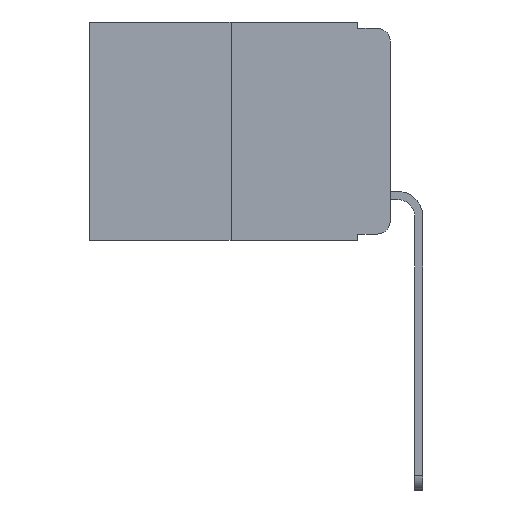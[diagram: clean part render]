
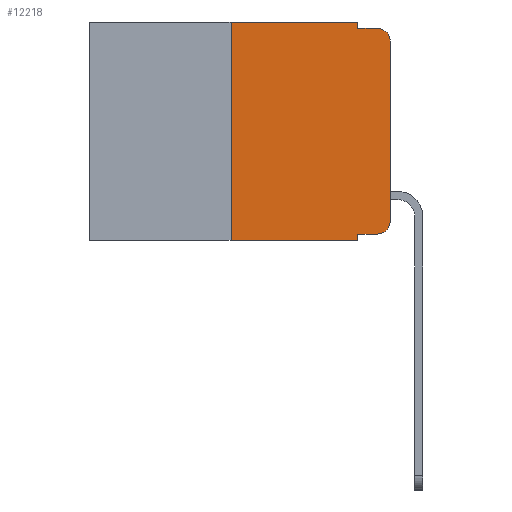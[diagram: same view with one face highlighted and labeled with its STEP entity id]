
A CAD part, left-side view. The second image highlights one B-rep face of the part: STEP entity #12218.
In plain terms, the highlighted planar face has unit normal (-1, 0, 0).
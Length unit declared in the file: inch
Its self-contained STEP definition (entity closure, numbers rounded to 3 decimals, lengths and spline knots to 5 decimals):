
#92 = CARTESIAN_POINT ( 'NONE',  ( 0., 0.25, -0.343 ) ) ;
#137 = VERTEX_POINT ( 'NONE', #10585 ) ;
#212 = EDGE_CURVE ( 'NONE', #8192, #11914, #12393, .T. ) ;
#644 = ORIENTED_EDGE ( 'NONE', *, *, #1718, .F. ) ;
#750 = CIRCLE ( 'NONE', #8688, 0.02 ) ;
#809 = DIRECTION ( 'NONE',  ( 0., 0., -1. ) ) ;
#830 = LINE ( 'NONE', #10785, #11550 ) ;
#1185 = CARTESIAN_POINT ( 'NONE',  ( 0., 0.051, -0.01 ) ) ;
#1364 = ORIENTED_EDGE ( 'NONE', *, *, #6208, .T. ) ;
#1379 = CARTESIAN_POINT ( 'NONE',  ( 0., 0.051, -0.333 ) ) ;
#1653 = EDGE_CURVE ( 'NONE', #8192, #5656, #4548, .T. ) ;
#1718 = EDGE_CURVE ( 'NONE', #12948, #137, #2515, .T. ) ;
#1779 = EDGE_CURVE ( 'NONE', #12948, #11914, #5555, .T. ) ;
#1780 = LINE ( 'NONE', #13300, #13002 ) ;
#2081 = EDGE_CURVE ( 'NONE', #5454, #8555, #10981, .T. ) ;
#2210 = ORIENTED_EDGE ( 'NONE', *, *, #2878, .T. ) ;
#2274 = DIRECTION ( 'NONE',  ( 0., -1., 0. ) ) ;
#2314 = ORIENTED_EDGE ( 'NONE', *, *, #1653, .T. ) ;
#2515 = LINE ( 'NONE', #4345, #10824 ) ;
#2773 = CARTESIAN_POINT ( 'NONE',  ( 0., 0.02, -0.01 ) ) ;
#2878 = EDGE_CURVE ( 'NONE', #9328, #3279, #750, .T. ) ;
#2961 = EDGE_CURVE ( 'NONE', #5656, #3837, #5689, .T. ) ;
#3122 = AXIS2_PLACEMENT_3D ( 'NONE', #7548, #4167, #13949 ) ;
#3279 = VERTEX_POINT ( 'NONE', #2773 ) ;
#3567 = CARTESIAN_POINT ( 'NONE',  ( 0., 0.473, 0. ) ) ;
#3784 = LINE ( 'NONE', #3567, #4441 ) ;
#3796 = ORIENTED_EDGE ( 'NONE', *, *, #2081, .F. ) ;
#3808 = CARTESIAN_POINT ( 'NONE',  ( 0., 0., -0.313 ) ) ;
#3837 = VERTEX_POINT ( 'NONE', #3808 ) ;
#4007 = DIRECTION ( 'NONE',  ( -1., 0., 0. ) ) ;
#4167 = DIRECTION ( 'NONE',  ( 1., 0., 0. ) ) ;
#4345 = CARTESIAN_POINT ( 'NONE',  ( 0., 0.25, 0. ) ) ;
#4377 = CARTESIAN_POINT ( 'NONE',  ( 0., 0.02, -0.333 ) ) ;
#4441 = VECTOR ( 'NONE', #5489, 39.37008 ) ;
#4459 = CARTESIAN_POINT ( 'NONE',  ( 0., 0.051, 0. ) ) ;
#4548 = LINE ( 'NONE', #13065, #8804 ) ;
#5315 = DIRECTION ( 'NONE',  ( 0., 0., -1. ) ) ;
#5454 = VERTEX_POINT ( 'NONE', #8460 ) ;
#5489 = DIRECTION ( 'NONE',  ( 0., -1., 0. ) ) ;
#5555 = LINE ( 'NONE', #11897, #7950 ) ;
#5656 = VERTEX_POINT ( 'NONE', #4377 ) ;
#5689 = CIRCLE ( 'NONE', #11594, 0.02 ) ;
#6059 = EDGE_CURVE ( 'NONE', #137, #5454, #3784, .T. ) ;
#6208 = EDGE_CURVE ( 'NONE', #3837, #9328, #830, .T. ) ;
#6386 = DIRECTION ( 'NONE',  ( -1., 0., 0. ) ) ;
#6430 = DIRECTION ( 'NONE',  ( 0., 0., 1. ) ) ;
#6542 = DIRECTION ( 'NONE',  ( 0., -1., 0. ) ) ;
#6680 = DIRECTION ( 'NONE',  ( 0., -1., 0. ) ) ;
#7548 = CARTESIAN_POINT ( 'NONE',  ( 0., 0.473, 0. ) ) ;
#7591 = EDGE_LOOP ( 'NONE', ( #1364, #2210, #13489, #3796, #13016, #644, #11150, #10753, #2314, #8291 ) ) ;
#7795 = DIRECTION ( 'NONE',  ( 0., 0., -1. ) ) ;
#7950 = VECTOR ( 'NONE', #2274, 39.37008 ) ;
#7951 = CARTESIAN_POINT ( 'NONE',  ( 0., 0., -0.03 ) ) ;
#8192 = VERTEX_POINT ( 'NONE', #1379 ) ;
#8291 = ORIENTED_EDGE ( 'NONE', *, *, #2961, .T. ) ;
#8460 = CARTESIAN_POINT ( 'NONE',  ( 0., 0.051, 0. ) ) ;
#8555 = VERTEX_POINT ( 'NONE', #1185 ) ;
#8688 = AXIS2_PLACEMENT_3D ( 'NONE', #12596, #4007, #809 ) ;
#8804 = VECTOR ( 'NONE', #6542, 39.37008 ) ;
#9328 = VERTEX_POINT ( 'NONE', #7951 ) ;
#9634 = CARTESIAN_POINT ( 'NONE',  ( 0., 0.02, -0.313 ) ) ;
#9770 = PLANE ( 'NONE',  #3122 ) ;
#9882 = FACE_OUTER_BOUND ( 'NONE', #7591, .T. ) ;
#9885 = EDGE_CURVE ( 'NONE', #8555, #3279, #1780, .T. ) ;
#10501 = DIRECTION ( 'NONE',  ( 0., 0., -1. ) ) ;
#10533 = DIRECTION ( 'NONE',  ( 0., 0., 1. ) ) ;
#10585 = CARTESIAN_POINT ( 'NONE',  ( 0., 0.25, 0. ) ) ;
#10753 = ORIENTED_EDGE ( 'NONE', *, *, #212, .F. ) ;
#10778 = CARTESIAN_POINT ( 'NONE',  ( 0., 0.051, 0. ) ) ;
#10785 = CARTESIAN_POINT ( 'NONE',  ( 0., 0., 0. ) ) ;
#10824 = VECTOR ( 'NONE', #6430, 39.37008 ) ;
#10981 = LINE ( 'NONE', #4459, #13877 ) ;
#11150 = ORIENTED_EDGE ( 'NONE', *, *, #1779, .T. ) ;
#11550 = VECTOR ( 'NONE', #10533, 39.37008 ) ;
#11594 = AXIS2_PLACEMENT_3D ( 'NONE', #9634, #6386, #10501 ) ;
#11897 = CARTESIAN_POINT ( 'NONE',  ( 0., 0.473, -0.343 ) ) ;
#11914 = VERTEX_POINT ( 'NONE', #13781 ) ;
#12218 = ADVANCED_FACE ( 'NONE', ( #9882 ), #9770, .F. ) ;
#12393 = LINE ( 'NONE', #10778, #13437 ) ;
#12596 = CARTESIAN_POINT ( 'NONE',  ( 0., 0.02, -0.03 ) ) ;
#12948 = VERTEX_POINT ( 'NONE', #92 ) ;
#13002 = VECTOR ( 'NONE', #6680, 39.37008 ) ;
#13016 = ORIENTED_EDGE ( 'NONE', *, *, #6059, .F. ) ;
#13065 = CARTESIAN_POINT ( 'NONE',  ( 0., 0.051, -0.333 ) ) ;
#13300 = CARTESIAN_POINT ( 'NONE',  ( 0., 0.051, -0.01 ) ) ;
#13437 = VECTOR ( 'NONE', #5315, 39.37008 ) ;
#13489 = ORIENTED_EDGE ( 'NONE', *, *, #9885, .F. ) ;
#13781 = CARTESIAN_POINT ( 'NONE',  ( 0., 0.051, -0.343 ) ) ;
#13877 = VECTOR ( 'NONE', #7795, 39.37008 ) ;
#13949 = DIRECTION ( 'NONE',  ( 0., 0., -1. ) ) ;
